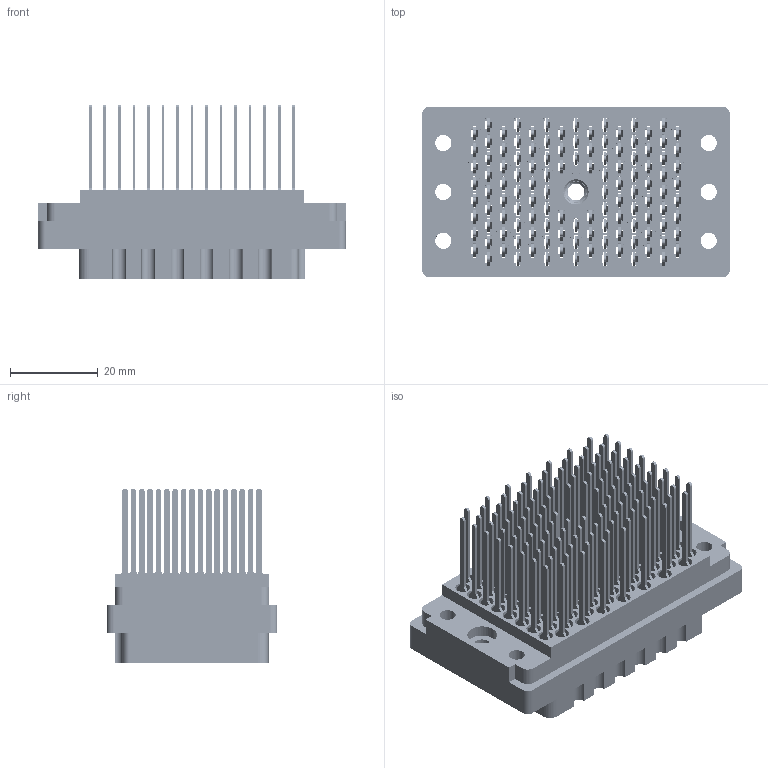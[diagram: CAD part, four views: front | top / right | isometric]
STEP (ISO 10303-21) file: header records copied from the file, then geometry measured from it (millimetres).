
FILE_DESCRIPTION (( 'STEP AP203' ), '1' );
FILE_NAME ('516-120-542-406.STEP', '2020-03-07T04:18:48', ( '' ), ( '' ), 'SwSTEP 2.0', 'SolidWorks 2016', '' );
FILE_SCHEMA (( 'CONFIG_CONTROL_DESIGN' ));
Length unit declared in the file: inch
Products named in the file (4): 516-120-542-406; 516-252-095-100; 516 Part Receptacle_120; 516-292-001_542 Contact
Assembly tree (122 placements, depth 2):
  516-120-542-406
    516 Part Receptacle_120
    516-292-001_542 Contact  x120
    516-252-095-100
Bounding box: 69.85 x 38.73 x 39.7 mm (x, y, z)
Volume: 30385.3 mm3; surface area: 64999.5 mm2
Topology: 122 solids, 122 shells, 11177 faces, 32493 edges, 21579 vertices
Faces by surface type: plane 6842, cylinder 3597, bspline 726, cone 12
Entity records: 94167 total; most frequent: CARTESIAN_POINT 17921, ORIENTED_EDGE 15482, DIRECTION 15048, EDGE_CURVE 7741, VECTOR 5714, LINE 5714, VERTEX_POINT 5157, AXIS2_PLACEMENT_3D 4667
